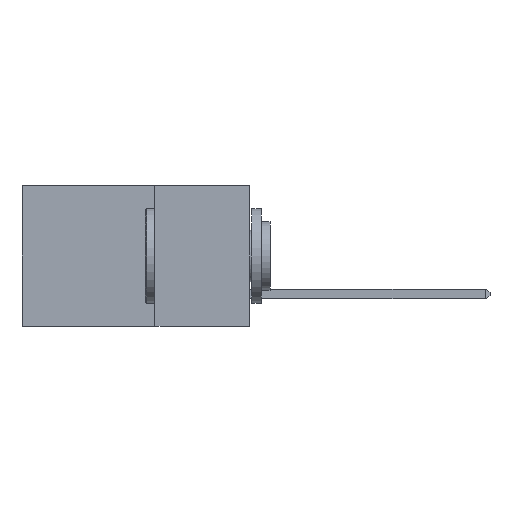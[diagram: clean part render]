
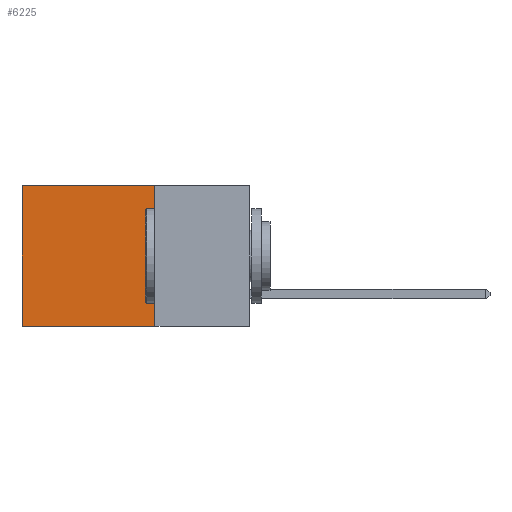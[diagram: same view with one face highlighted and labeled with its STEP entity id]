
A CAD part, left-side view. The second image highlights one B-rep face of the part: STEP entity #6225.
In plain terms, the highlighted planar face has unit normal (-1, 0, 0).
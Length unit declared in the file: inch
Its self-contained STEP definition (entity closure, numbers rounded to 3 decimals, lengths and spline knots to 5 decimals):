
#72 = CARTESIAN_POINT ( 'NONE',  ( 0.2875, 0.25, -0.37 ) ) ;
#561 = AXIS2_PLACEMENT_3D ( 'NONE', #10357, #4185, #11344 ) ;
#1617 = VERTEX_POINT ( 'NONE', #9973 ) ;
#1653 = EDGE_CURVE ( 'NONE', #1617, #12860, #10259, .T. ) ;
#2340 = DIRECTION ( 'NONE',  ( 0., 0., -1. ) ) ;
#2836 = CARTESIAN_POINT ( 'NONE',  ( 0.2875, 0.6, 0. ) ) ;
#3020 = CARTESIAN_POINT ( 'NONE',  ( 0.2875, 0.25, 0. ) ) ;
#3121 = PLANE ( 'NONE',  #561 ) ;
#3641 = LINE ( 'NONE', #12969, #8539 ) ;
#3798 = ORIENTED_EDGE ( 'NONE', *, *, #9258, .T. ) ;
#4185 = DIRECTION ( 'NONE',  ( 1., 0., 0. ) ) ;
#4596 = VECTOR ( 'NONE', #5198, 39.37008 ) ;
#5198 = DIRECTION ( 'NONE',  ( 0., 1., 0. ) ) ;
#5617 = ORIENTED_EDGE ( 'NONE', *, *, #9458, .T. ) ;
#6225 = ADVANCED_FACE ( 'NONE', ( #12353 ), #3121, .F. ) ;
#6713 = EDGE_CURVE ( 'NONE', #12860, #12103, #3641, .T. ) ;
#7520 = VECTOR ( 'NONE', #2340, 39.37008 ) ;
#7597 = CARTESIAN_POINT ( 'NONE',  ( 0.2875, 0.6, 0. ) ) ;
#8027 = EDGE_LOOP ( 'NONE', ( #5617, #9007, #11632, #3798 ) ) ;
#8533 = CARTESIAN_POINT ( 'NONE',  ( 0.2875, 0.25, 0. ) ) ;
#8539 = VECTOR ( 'NONE', #10133, 39.37008 ) ;
#8542 = DIRECTION ( 'NONE',  ( 0., 0., -1. ) ) ;
#9007 = ORIENTED_EDGE ( 'NONE', *, *, #6713, .F. ) ;
#9258 = EDGE_CURVE ( 'NONE', #1617, #11410, #12576, .T. ) ;
#9458 = EDGE_CURVE ( 'NONE', #11410, #12103, #12711, .T. ) ;
#9973 = CARTESIAN_POINT ( 'NONE',  ( 0.2875, 0.25, 0. ) ) ;
#10133 = DIRECTION ( 'NONE',  ( 0., 1., 0. ) ) ;
#10259 = LINE ( 'NONE', #8533, #12193 ) ;
#10357 = CARTESIAN_POINT ( 'NONE',  ( 0.2875, 0.25, 0. ) ) ;
#11344 = DIRECTION ( 'NONE',  ( 0., 0., -1. ) ) ;
#11410 = VERTEX_POINT ( 'NONE', #2836 ) ;
#11632 = ORIENTED_EDGE ( 'NONE', *, *, #1653, .F. ) ;
#12103 = VERTEX_POINT ( 'NONE', #12959 ) ;
#12193 = VECTOR ( 'NONE', #8542, 39.37008 ) ;
#12353 = FACE_OUTER_BOUND ( 'NONE', #8027, .T. ) ;
#12576 = LINE ( 'NONE', #3020, #4596 ) ;
#12711 = LINE ( 'NONE', #7597, #7520 ) ;
#12860 = VERTEX_POINT ( 'NONE', #72 ) ;
#12959 = CARTESIAN_POINT ( 'NONE',  ( 0.2875, 0.6, -0.37 ) ) ;
#12969 = CARTESIAN_POINT ( 'NONE',  ( 0.2875, 0.25, -0.37 ) ) ;
